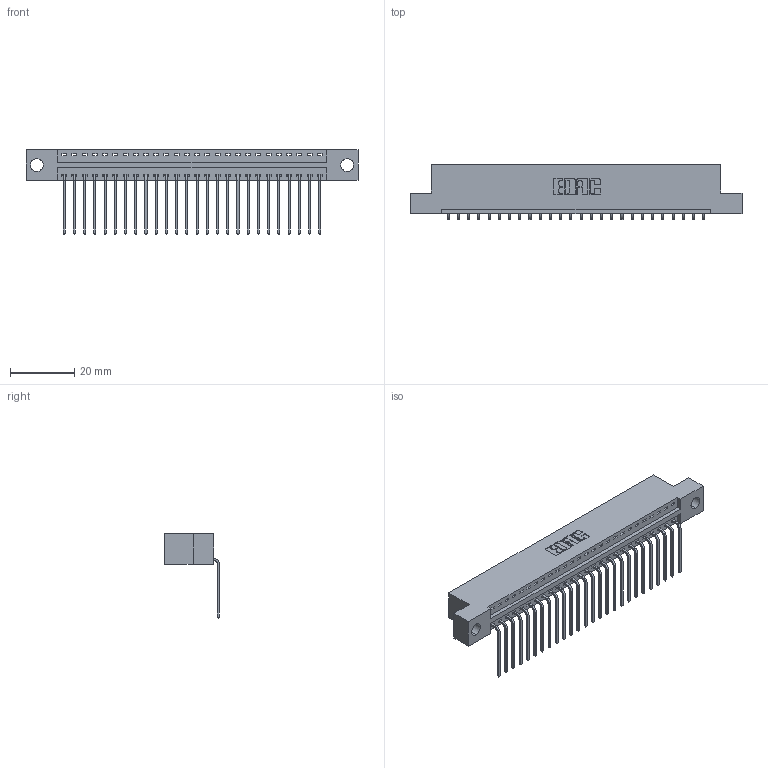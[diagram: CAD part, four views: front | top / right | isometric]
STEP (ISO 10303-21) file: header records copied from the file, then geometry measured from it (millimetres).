
FILE_DESCRIPTION (( 'STEP AP203' ), '1' );
FILE_NAME ('346-026-559-104.STEP', '2022-05-06T03:34:20', ( '' ), ( '' ), 'SwSTEP 2.0', 'SolidWorks 2020', '' );
FILE_SCHEMA (( 'CONFIG_CONTROL_DESIGN' ));
Length unit declared in the file: inch
Products named in the file (3): 346-026-559-104; 346 Part_Flush Mounting Lugs - 0.156 Dia-TH; 345-292-001_558 559 Tail - 1
Assembly tree (27 placements, depth 2):
  346-026-559-104
    346 Part_Flush Mounting Lugs - 0.156 Dia-TH
    345-292-001_558 559 Tail - 1  x26
Bounding box: 103.12 x 17.08 x 26.16 mm (x, y, z)
Volume: 9741.7 mm3; surface area: 12357.2 mm2
Topology: 27 solids, 27 shells, 1696 faces, 5097 edges, 3362 vertices
Faces by surface type: plane 1182, cylinder 514
Entity records: 18793 total; most frequent: CARTESIAN_POINT 3236, ORIENTED_EDGE 3194, DIRECTION 2873, EDGE_CURVE 1597, VECTOR 1361, LINE 1361, VERTEX_POINT 1062, AXIS2_PLACEMENT_3D 756
